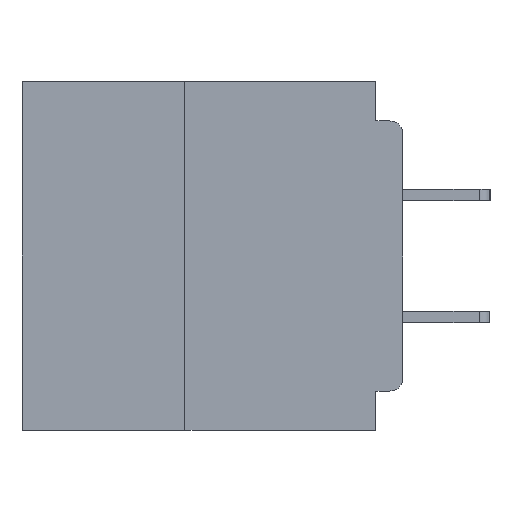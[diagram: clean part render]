
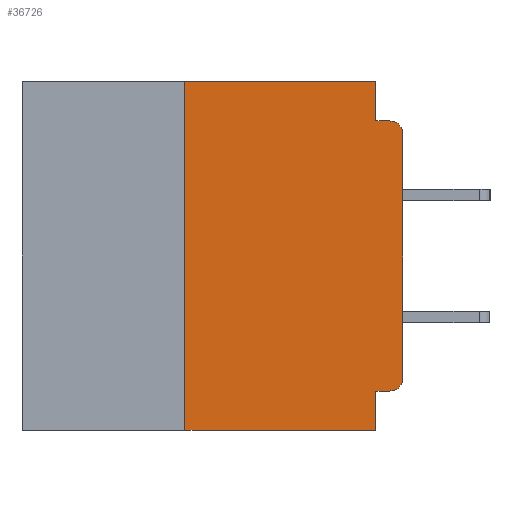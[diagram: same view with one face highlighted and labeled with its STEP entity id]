
A CAD part, left-side view. The second image highlights one B-rep face of the part: STEP entity #36726.
In plain terms, the highlighted planar face has unit normal (-1, 0, 0).
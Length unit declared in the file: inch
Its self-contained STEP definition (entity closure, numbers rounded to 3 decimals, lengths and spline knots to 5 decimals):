
#159 = VERTEX_POINT ( 'NONE', #47620 ) ;
#1655 = VERTEX_POINT ( 'NONE', #2360 ) ;
#1679 = VECTOR ( 'NONE', #11630, 39.37008 ) ;
#1730 = CARTESIAN_POINT ( 'NONE',  ( 0., 0.25, -0.4 ) ) ;
#1980 = DIRECTION ( 'NONE',  ( 0., 0., -1. ) ) ;
#2360 = CARTESIAN_POINT ( 'NONE',  ( 0., 0.015, -0.355 ) ) ;
#2572 = AXIS2_PLACEMENT_3D ( 'NONE', #26752, #3008, #30759 ) ;
#2934 = LINE ( 'NONE', #43233, #1679 ) ;
#3008 = DIRECTION ( 'NONE',  ( 1., 0., 0. ) ) ;
#3238 = DIRECTION ( 'NONE',  ( 0., -1., 0. ) ) ;
#3457 = ORIENTED_EDGE ( 'NONE', *, *, #7015, .T. ) ;
#4289 = ORIENTED_EDGE ( 'NONE', *, *, #31689, .F. ) ;
#4432 = VECTOR ( 'NONE', #3238, 39.37008 ) ;
#5279 = LINE ( 'NONE', #48297, #46049 ) ;
#5720 = EDGE_CURVE ( 'NONE', #25437, #10589, #5279, .T. ) ;
#5751 = CARTESIAN_POINT ( 'NONE',  ( 0., 0.25, 0. ) ) ;
#5862 = CARTESIAN_POINT ( 'NONE',  ( 0., 0.031, -0.355 ) ) ;
#6181 = CIRCLE ( 'NONE', #39443, 0.015 ) ;
#7015 = EDGE_CURVE ( 'NONE', #15237, #159, #25535, .T. ) ;
#7365 = VERTEX_POINT ( 'NONE', #39502 ) ;
#7905 = EDGE_CURVE ( 'NONE', #7365, #10589, #18648, .T. ) ;
#8563 = ORIENTED_EDGE ( 'NONE', *, *, #41654, .F. ) ;
#9323 = DIRECTION ( 'NONE',  ( 0., 0., 1. ) ) ;
#9359 = EDGE_LOOP ( 'NONE', ( #23318, #3457, #8563, #33346, #45011, #17929, #12344, #50615, #4289, #9404 ) ) ;
#9404 = ORIENTED_EDGE ( 'NONE', *, *, #12878, .T. ) ;
#9752 = CARTESIAN_POINT ( 'NONE',  ( 0., 0.031, -0.045 ) ) ;
#9937 = VECTOR ( 'NONE', #51222, 39.37008 ) ;
#10121 = DIRECTION ( 'NONE',  ( -1., 0., 0. ) ) ;
#10589 = VERTEX_POINT ( 'NONE', #36118 ) ;
#11630 = DIRECTION ( 'NONE',  ( 0., -1., 0. ) ) ;
#12344 = ORIENTED_EDGE ( 'NONE', *, *, #7905, .T. ) ;
#12878 = EDGE_CURVE ( 'NONE', #1655, #13921, #6181, .T. ) ;
#12995 = DIRECTION ( 'NONE',  ( 0., 0., -1. ) ) ;
#13921 = VERTEX_POINT ( 'NONE', #48698 ) ;
#15237 = VERTEX_POINT ( 'NONE', #33156 ) ;
#17929 = ORIENTED_EDGE ( 'NONE', *, *, #20530, .F. ) ;
#18648 = LINE ( 'NONE', #50224, #38430 ) ;
#19381 = VECTOR ( 'NONE', #45127, 39.37008 ) ;
#20530 = EDGE_CURVE ( 'NONE', #7365, #48820, #40360, .T. ) ;
#23318 = ORIENTED_EDGE ( 'NONE', *, *, #40851, .T. ) ;
#25437 = VERTEX_POINT ( 'NONE', #5862 ) ;
#25535 = CIRCLE ( 'NONE', #26186, 0.015 ) ;
#25754 = DIRECTION ( 'NONE',  ( -1., 0., 0. ) ) ;
#25870 = CARTESIAN_POINT ( 'NONE',  ( 0., 0., -0.355 ) ) ;
#26186 = AXIS2_PLACEMENT_3D ( 'NONE', #33822, #10121, #37817 ) ;
#26752 = CARTESIAN_POINT ( 'NONE',  ( 0., 0.437, 0. ) ) ;
#28921 = VERTEX_POINT ( 'NONE', #9752 ) ;
#29843 = DIRECTION ( 'NONE',  ( 0., 1., 0. ) ) ;
#30759 = DIRECTION ( 'NONE',  ( 0., 0., -1. ) ) ;
#31689 = EDGE_CURVE ( 'NONE', #1655, #25437, #34963, .T. ) ;
#33156 = CARTESIAN_POINT ( 'NONE',  ( 0., 0., -0.06 ) ) ;
#33346 = ORIENTED_EDGE ( 'NONE', *, *, #44520, .F. ) ;
#33470 = LINE ( 'NONE', #47259, #9937 ) ;
#33662 = VERTEX_POINT ( 'NONE', #39766 ) ;
#33822 = CARTESIAN_POINT ( 'NONE',  ( 0., 0.015, -0.06 ) ) ;
#34554 = PLANE ( 'NONE',  #2572 ) ;
#34943 = CARTESIAN_POINT ( 'NONE',  ( 0., 0., -0.045 ) ) ;
#34963 = LINE ( 'NONE', #25870, #42947 ) ;
#35452 = LINE ( 'NONE', #36997, #42188 ) ;
#36118 = CARTESIAN_POINT ( 'NONE',  ( 0., 0.031, -0.4 ) ) ;
#36726 = ADVANCED_FACE ( 'NONE', ( #44474 ), #34554, .F. ) ;
#36997 = CARTESIAN_POINT ( 'NONE',  ( 0., 0., 0. ) ) ;
#37817 = DIRECTION ( 'NONE',  ( 0., 0., -1. ) ) ;
#38424 = DIRECTION ( 'NONE',  ( 0., -1., 0. ) ) ;
#38430 = VECTOR ( 'NONE', #38424, 39.37008 ) ;
#39443 = AXIS2_PLACEMENT_3D ( 'NONE', #49305, #25754, #1980 ) ;
#39502 = CARTESIAN_POINT ( 'NONE',  ( 0., 0.25, -0.4 ) ) ;
#39766 = CARTESIAN_POINT ( 'NONE',  ( 0., 0.031, 0. ) ) ;
#40360 = LINE ( 'NONE', #1730, #19381 ) ;
#40851 = EDGE_CURVE ( 'NONE', #13921, #15237, #35452, .T. ) ;
#41654 = EDGE_CURVE ( 'NONE', #28921, #159, #45229, .T. ) ;
#42188 = VECTOR ( 'NONE', #9323, 39.37008 ) ;
#42947 = VECTOR ( 'NONE', #29843, 39.37008 ) ;
#43233 = CARTESIAN_POINT ( 'NONE',  ( 0., 0.437, 0. ) ) ;
#44474 = FACE_OUTER_BOUND ( 'NONE', #9359, .T. ) ;
#44520 = EDGE_CURVE ( 'NONE', #33662, #28921, #33470, .T. ) ;
#45011 = ORIENTED_EDGE ( 'NONE', *, *, #45723, .F. ) ;
#45127 = DIRECTION ( 'NONE',  ( 0., 0., 1. ) ) ;
#45229 = LINE ( 'NONE', #34943, #4432 ) ;
#45723 = EDGE_CURVE ( 'NONE', #48820, #33662, #2934, .T. ) ;
#46049 = VECTOR ( 'NONE', #12995, 39.37008 ) ;
#47259 = CARTESIAN_POINT ( 'NONE',  ( 0., 0.031, 0. ) ) ;
#47620 = CARTESIAN_POINT ( 'NONE',  ( 0., 0.015, -0.045 ) ) ;
#48297 = CARTESIAN_POINT ( 'NONE',  ( 0., 0.031, -0.4 ) ) ;
#48698 = CARTESIAN_POINT ( 'NONE',  ( 0., 0., -0.34 ) ) ;
#48820 = VERTEX_POINT ( 'NONE', #5751 ) ;
#49305 = CARTESIAN_POINT ( 'NONE',  ( 0., 0.015, -0.34 ) ) ;
#50224 = CARTESIAN_POINT ( 'NONE',  ( 0., 0.437, -0.4 ) ) ;
#50615 = ORIENTED_EDGE ( 'NONE', *, *, #5720, .F. ) ;
#51222 = DIRECTION ( 'NONE',  ( 0., 0., -1. ) ) ;
